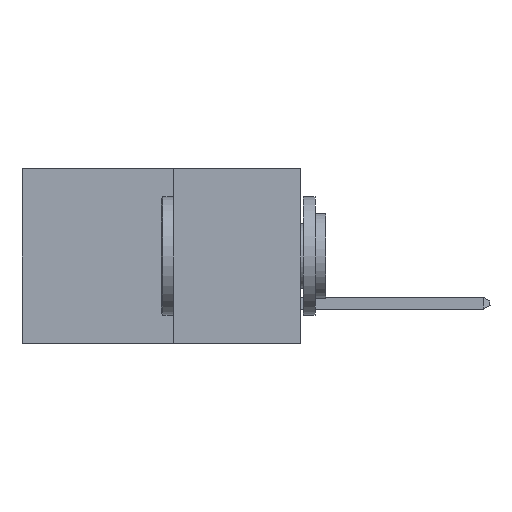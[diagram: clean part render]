
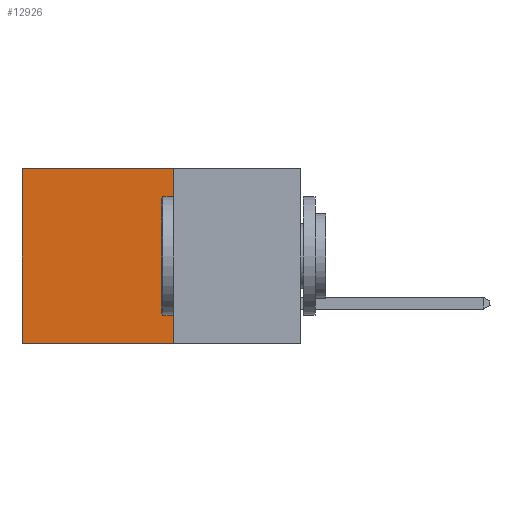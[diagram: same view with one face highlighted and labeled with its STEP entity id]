
A CAD part, left-side view. The second image highlights one B-rep face of the part: STEP entity #12926.
In plain terms, the highlighted planar face has unit normal (-1, 0, 0).
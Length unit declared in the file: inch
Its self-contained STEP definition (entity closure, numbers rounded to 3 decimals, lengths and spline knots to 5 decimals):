
#280 = EDGE_CURVE ( 'NONE', #7717, #10308, #10150, .T. ) ;
#412 = VECTOR ( 'NONE', #10668, 39.37008 ) ;
#563 = PLANE ( 'NONE',  #4855 ) ;
#1228 = EDGE_CURVE ( 'NONE', #10308, #10338, #12531, .T. ) ;
#4855 = AXIS2_PLACEMENT_3D ( 'NONE', #13918, #5091, #15364 ) ;
#5091 = DIRECTION ( 'NONE',  ( 1., 0., 0. ) ) ;
#5688 = VERTEX_POINT ( 'NONE', #13676 ) ;
#6203 = VECTOR ( 'NONE', #17757, 39.37008 ) ;
#7717 = VERTEX_POINT ( 'NONE', #10589 ) ;
#8274 = LINE ( 'NONE', #16547, #412 ) ;
#8817 = CARTESIAN_POINT ( 'NONE',  ( 0.277, 0.59, -0.37 ) ) ;
#9030 = CARTESIAN_POINT ( 'NONE',  ( 0.277, 0.27, 0. ) ) ;
#10041 = CARTESIAN_POINT ( 'NONE',  ( 0.277, 0.27, -0.37 ) ) ;
#10150 = LINE ( 'NONE', #10041, #14044 ) ;
#10308 = VERTEX_POINT ( 'NONE', #14718 ) ;
#10338 = VERTEX_POINT ( 'NONE', #8817 ) ;
#10354 = EDGE_LOOP ( 'NONE', ( #18757, #11486, #12077, #17957 ) ) ;
#10589 = CARTESIAN_POINT ( 'NONE',  ( 0.277, 0.27, 0. ) ) ;
#10668 = DIRECTION ( 'NONE',  ( 0., 0., -1. ) ) ;
#11486 = ORIENTED_EDGE ( 'NONE', *, *, #1228, .F. ) ;
#12077 = ORIENTED_EDGE ( 'NONE', *, *, #280, .F. ) ;
#12109 = EDGE_CURVE ( 'NONE', #7717, #5688, #17877, .T. ) ;
#12531 = LINE ( 'NONE', #17502, #16369 ) ;
#12926 = ADVANCED_FACE ( 'NONE', ( #14280 ), #563, .F. ) ;
#13676 = CARTESIAN_POINT ( 'NONE',  ( 0.277, 0.59, 0. ) ) ;
#13918 = CARTESIAN_POINT ( 'NONE',  ( 0.277, 0.27, -0.37 ) ) ;
#14044 = VECTOR ( 'NONE', #15724, 39.37008 ) ;
#14280 = FACE_OUTER_BOUND ( 'NONE', #10354, .T. ) ;
#14718 = CARTESIAN_POINT ( 'NONE',  ( 0.277, 0.27, -0.37 ) ) ;
#15364 = DIRECTION ( 'NONE',  ( 0., 0., -1. ) ) ;
#15724 = DIRECTION ( 'NONE',  ( 0., 0., -1. ) ) ;
#16369 = VECTOR ( 'NONE', #17299, 39.37008 ) ;
#16547 = CARTESIAN_POINT ( 'NONE',  ( 0.277, 0.59, -0.37 ) ) ;
#17299 = DIRECTION ( 'NONE',  ( 0., 1., 0. ) ) ;
#17502 = CARTESIAN_POINT ( 'NONE',  ( 0.277, 0.27, -0.37 ) ) ;
#17757 = DIRECTION ( 'NONE',  ( 0., 1., 0. ) ) ;
#17877 = LINE ( 'NONE', #9030, #6203 ) ;
#17921 = EDGE_CURVE ( 'NONE', #5688, #10338, #8274, .T. ) ;
#17957 = ORIENTED_EDGE ( 'NONE', *, *, #12109, .T. ) ;
#18757 = ORIENTED_EDGE ( 'NONE', *, *, #17921, .T. ) ;
